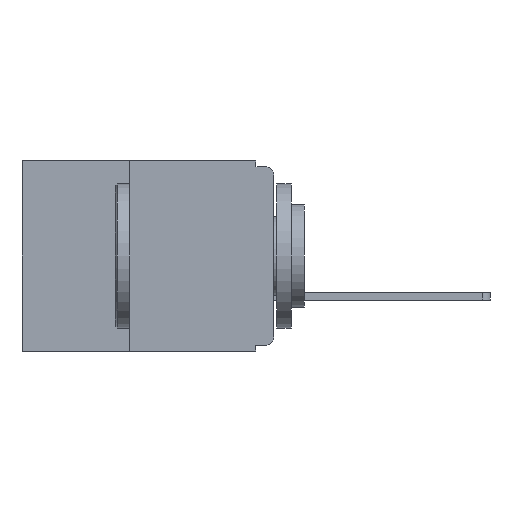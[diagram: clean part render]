
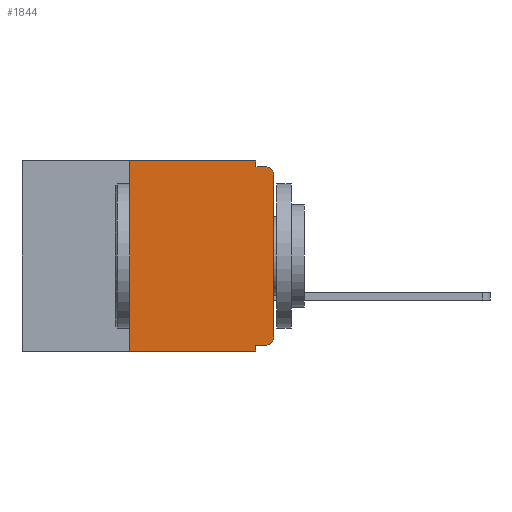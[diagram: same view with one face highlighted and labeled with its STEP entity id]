
A CAD part, left-side view. The second image highlights one B-rep face of the part: STEP entity #1844.
In plain terms, the highlighted planar face has unit normal (-1, 0, 0).
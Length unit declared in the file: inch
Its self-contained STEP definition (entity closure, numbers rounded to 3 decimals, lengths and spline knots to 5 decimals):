
#31 = DIRECTION ( 'NONE',  ( 0., 0., 1. ) ) ;
#235 = CARTESIAN_POINT ( 'NONE',  ( 0., 0.25, -0.33 ) ) ;
#636 = AXIS2_PLACEMENT_3D ( 'NONE', #12607, #12693, #17232 ) ;
#786 = DIRECTION ( 'NONE',  ( 0., 0., -1. ) ) ;
#806 = DIRECTION ( 'NONE',  ( -1., 0., 0. ) ) ;
#860 = VECTOR ( 'NONE', #5084, 39.37008 ) ;
#893 = CARTESIAN_POINT ( 'NONE',  ( 0., 0.25, -0.33 ) ) ;
#933 = CARTESIAN_POINT ( 'NONE',  ( 0., 0.015, -0.025 ) ) ;
#969 = LINE ( 'NONE', #4332, #860 ) ;
#1292 = VERTEX_POINT ( 'NONE', #1465 ) ;
#1322 = CARTESIAN_POINT ( 'NONE',  ( 0., 0.031, -0.32 ) ) ;
#1465 = CARTESIAN_POINT ( 'NONE',  ( 0., 0.25, 0. ) ) ;
#1844 = ADVANCED_FACE ( 'NONE', ( #4863 ), #13266, .F. ) ;
#2513 = CARTESIAN_POINT ( 'NONE',  ( 0., 0., -0.305 ) ) ;
#2780 = CARTESIAN_POINT ( 'NONE',  ( 0., 0.031, -0.33 ) ) ;
#3755 = VECTOR ( 'NONE', #16564, 39.37008 ) ;
#3774 = LINE ( 'NONE', #2780, #3755 ) ;
#3955 = EDGE_CURVE ( 'NONE', #14312, #14033, #8061, .T. ) ;
#4332 = CARTESIAN_POINT ( 'NONE',  ( 0., 0.437, 0. ) ) ;
#4337 = VECTOR ( 'NONE', #10090, 39.37008 ) ;
#4483 = LINE ( 'NONE', #10613, #4337 ) ;
#4722 = CARTESIAN_POINT ( 'NONE',  ( 0., 0.031, -0.01 ) ) ;
#4761 = VERTEX_POINT ( 'NONE', #1322 ) ;
#4863 = FACE_OUTER_BOUND ( 'NONE', #10438, .T. ) ;
#4942 = CIRCLE ( 'NONE', #8360, 0.015 ) ;
#5084 = DIRECTION ( 'NONE',  ( 0., -1., 0. ) ) ;
#5098 = VECTOR ( 'NONE', #11839, 39.37008 ) ;
#5179 = LINE ( 'NONE', #13438, #5098 ) ;
#5625 = VECTOR ( 'NONE', #31, 39.37008 ) ;
#5783 = LINE ( 'NONE', #235, #5625 ) ;
#6068 = VERTEX_POINT ( 'NONE', #15364 ) ;
#6722 = VECTOR ( 'NONE', #12388, 39.37008 ) ;
#6967 = LINE ( 'NONE', #13677, #6722 ) ;
#7659 = VERTEX_POINT ( 'NONE', #16960 ) ;
#8061 = CIRCLE ( 'NONE', #14257, 0.015 ) ;
#8360 = AXIS2_PLACEMENT_3D ( 'NONE', #933, #806, #786 ) ;
#8694 = VERTEX_POINT ( 'NONE', #893 ) ;
#9467 = VERTEX_POINT ( 'NONE', #10661 ) ;
#9482 = EDGE_CURVE ( 'NONE', #14033, #6068, #4483, .T. ) ;
#10090 = DIRECTION ( 'NONE',  ( 0., 0., 1. ) ) ;
#10304 = ORIENTED_EDGE ( 'NONE', *, *, #15763, .F. ) ;
#10345 = CARTESIAN_POINT ( 'NONE',  ( 0., 0., -0.32 ) ) ;
#10408 = CARTESIAN_POINT ( 'NONE',  ( 0., 0.015, -0.32 ) ) ;
#10438 = EDGE_LOOP ( 'NONE', ( #13184, #13536, #13884, #14064, #16563, #10304, #14569, #17166, #16301, #16599 ) ) ;
#10611 = EDGE_CURVE ( 'NONE', #1292, #9467, #969, .T. ) ;
#10613 = CARTESIAN_POINT ( 'NONE',  ( 0., 0., 0. ) ) ;
#10661 = CARTESIAN_POINT ( 'NONE',  ( 0., 0.031, 0. ) ) ;
#11267 = VECTOR ( 'NONE', #14841, 39.37008 ) ;
#11321 = LINE ( 'NONE', #14892, #11267 ) ;
#11423 = LINE ( 'NONE', #10345, #14539 ) ;
#11470 = DIRECTION ( 'NONE',  ( 0., 1., 0. ) ) ;
#11839 = DIRECTION ( 'NONE',  ( 0., -1., 0. ) ) ;
#12388 = DIRECTION ( 'NONE',  ( 0., 0., -1. ) ) ;
#12431 = EDGE_CURVE ( 'NONE', #6068, #16668, #4942, .T. ) ;
#12607 = CARTESIAN_POINT ( 'NONE',  ( 0., 0.437, 0. ) ) ;
#12693 = DIRECTION ( 'NONE',  ( 1., 0., 0. ) ) ;
#13184 = ORIENTED_EDGE ( 'NONE', *, *, #9482, .T. ) ;
#13266 = PLANE ( 'NONE',  #636 ) ;
#13438 = CARTESIAN_POINT ( 'NONE',  ( 0., 0.437, -0.33 ) ) ;
#13536 = ORIENTED_EDGE ( 'NONE', *, *, #12431, .T. ) ;
#13677 = CARTESIAN_POINT ( 'NONE',  ( 0., 0.031, 0. ) ) ;
#13884 = ORIENTED_EDGE ( 'NONE', *, *, #14694, .F. ) ;
#14033 = VERTEX_POINT ( 'NONE', #2513 ) ;
#14064 = ORIENTED_EDGE ( 'NONE', *, *, #15560, .F. ) ;
#14257 = AXIS2_PLACEMENT_3D ( 'NONE', #15827, #15764, #15750 ) ;
#14312 = VERTEX_POINT ( 'NONE', #10408 ) ;
#14539 = VECTOR ( 'NONE', #11470, 39.37008 ) ;
#14569 = ORIENTED_EDGE ( 'NONE', *, *, #15831, .T. ) ;
#14694 = EDGE_CURVE ( 'NONE', #17316, #16668, #11321, .T. ) ;
#14841 = DIRECTION ( 'NONE',  ( 0., -1., 0. ) ) ;
#14892 = CARTESIAN_POINT ( 'NONE',  ( 0., 0., -0.01 ) ) ;
#15364 = CARTESIAN_POINT ( 'NONE',  ( 0., 0., -0.025 ) ) ;
#15560 = EDGE_CURVE ( 'NONE', #9467, #17316, #6967, .T. ) ;
#15750 = DIRECTION ( 'NONE',  ( 0., 0., -1. ) ) ;
#15763 = EDGE_CURVE ( 'NONE', #8694, #1292, #5783, .T. ) ;
#15764 = DIRECTION ( 'NONE',  ( -1., 0., 0. ) ) ;
#15827 = CARTESIAN_POINT ( 'NONE',  ( 0., 0.015, -0.305 ) ) ;
#15831 = EDGE_CURVE ( 'NONE', #8694, #7659, #5179, .T. ) ;
#16080 = EDGE_CURVE ( 'NONE', #4761, #7659, #3774, .T. ) ;
#16301 = ORIENTED_EDGE ( 'NONE', *, *, #17614, .F. ) ;
#16563 = ORIENTED_EDGE ( 'NONE', *, *, #10611, .F. ) ;
#16564 = DIRECTION ( 'NONE',  ( 0., 0., -1. ) ) ;
#16599 = ORIENTED_EDGE ( 'NONE', *, *, #3955, .T. ) ;
#16668 = VERTEX_POINT ( 'NONE', #17420 ) ;
#16960 = CARTESIAN_POINT ( 'NONE',  ( 0., 0.031, -0.33 ) ) ;
#17166 = ORIENTED_EDGE ( 'NONE', *, *, #16080, .F. ) ;
#17232 = DIRECTION ( 'NONE',  ( 0., 0., -1. ) ) ;
#17316 = VERTEX_POINT ( 'NONE', #4722 ) ;
#17420 = CARTESIAN_POINT ( 'NONE',  ( 0., 0.015, -0.01 ) ) ;
#17614 = EDGE_CURVE ( 'NONE', #14312, #4761, #11423, .T. ) ;
